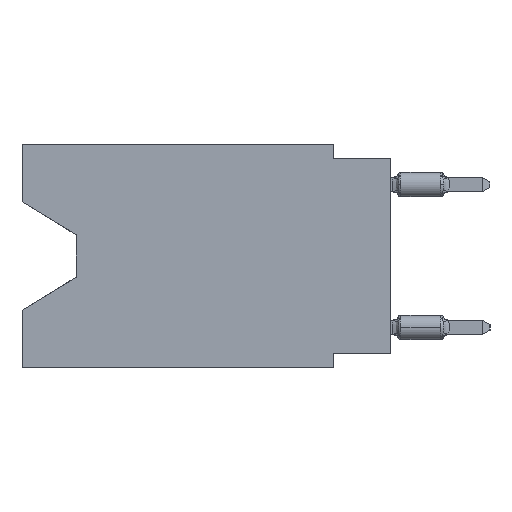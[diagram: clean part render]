
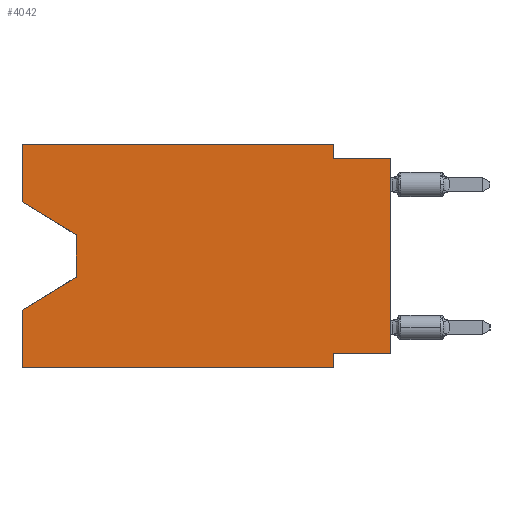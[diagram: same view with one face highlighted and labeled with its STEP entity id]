
A CAD part, left-side view. The second image highlights one B-rep face of the part: STEP entity #4042.
In plain terms, the highlighted planar face has unit normal (-1, 0, 0).
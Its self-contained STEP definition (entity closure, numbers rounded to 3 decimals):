
#632 = CARTESIAN_POINT ( 'NONE',  ( 0., 13.97, -4.013 ) ) ;
#1037 = VERTEX_POINT ( 'NONE', #12640 ) ;
#1064 = ORIENTED_EDGE ( 'NONE', *, *, #12744, .T. ) ;
#1403 = VECTOR ( 'NONE', #12382, 1000. ) ;
#1657 = LINE ( 'NONE', #27169, #15389 ) ;
#2208 = CARTESIAN_POINT ( 'NONE',  ( 0., 16.383, -7.36 ) ) ;
#2257 = VERTEX_POINT ( 'NONE', #24532 ) ;
#2273 = LINE ( 'NONE', #18485, #5044 ) ;
#2495 = VERTEX_POINT ( 'NONE', #13733 ) ;
#2797 = VERTEX_POINT ( 'NONE', #632 ) ;
#2970 = CARTESIAN_POINT ( 'NONE',  ( 0., 16.383, -2.546 ) ) ;
#3284 = VECTOR ( 'NONE', #19489, 1000. ) ;
#3533 = LINE ( 'NONE', #15798, #15662 ) ;
#3560 = DIRECTION ( 'NONE',  ( 0., 0., -1. ) ) ;
#3860 = CARTESIAN_POINT ( 'NONE',  ( 0., 2.54, -9.906 ) ) ;
#4042 = ADVANCED_FACE ( 'NONE', ( #20989 ), #18377, .F. ) ;
#4954 = CARTESIAN_POINT ( 'NONE',  ( 0., 16.383, 0. ) ) ;
#5044 = VECTOR ( 'NONE', #14252, 1000. ) ;
#5098 = CARTESIAN_POINT ( 'NONE',  ( 0., 13.97, -5.893 ) ) ;
#5673 = ORIENTED_EDGE ( 'NONE', *, *, #21150, .T. ) ;
#5781 = VECTOR ( 'NONE', #15855, 1000. ) ;
#6340 = EDGE_LOOP ( 'NONE', ( #1064, #19126, #24900, #10938, #5673, #23759, #12050, #23353, #22663, #14759, #27039, #16289 ) ) ;
#6469 = DIRECTION ( 'NONE',  ( 0., 0., 1. ) ) ;
#7064 = VECTOR ( 'NONE', #29134, 1000. ) ;
#7125 = VERTEX_POINT ( 'NONE', #28111 ) ;
#7310 = EDGE_CURVE ( 'NONE', #12395, #2495, #1657, .T. ) ;
#7480 = LINE ( 'NONE', #2970, #16596 ) ;
#8751 = CARTESIAN_POINT ( 'NONE',  ( 0., 16.383, 0. ) ) ;
#8922 = VERTEX_POINT ( 'NONE', #16013 ) ;
#9292 = DIRECTION ( 'NONE',  ( 0., 0., -1. ) ) ;
#10331 = VERTEX_POINT ( 'NONE', #26218 ) ;
#10938 = ORIENTED_EDGE ( 'NONE', *, *, #13830, .F. ) ;
#11026 = VECTOR ( 'NONE', #3560, 1000. ) ;
#11771 = CARTESIAN_POINT ( 'NONE',  ( 0., 16.383, -9.906 ) ) ;
#11910 = DIRECTION ( 'NONE',  ( 0., -0.855, -0.519 ) ) ;
#11912 = LINE ( 'NONE', #20569, #5781 ) ;
#11975 = VERTEX_POINT ( 'NONE', #26419 ) ;
#12050 = ORIENTED_EDGE ( 'NONE', *, *, #22576, .F. ) ;
#12124 = EDGE_CURVE ( 'NONE', #2257, #1037, #18767, .T. ) ;
#12382 = DIRECTION ( 'NONE',  ( 0., 0.855, -0.519 ) ) ;
#12395 = VERTEX_POINT ( 'NONE', #13130 ) ;
#12640 = CARTESIAN_POINT ( 'NONE',  ( 0., 2.54, 0. ) ) ;
#12718 = EDGE_CURVE ( 'NONE', #2797, #16454, #14493, .T. ) ;
#12744 = EDGE_CURVE ( 'NONE', #8922, #2797, #7480, .T. ) ;
#13130 = CARTESIAN_POINT ( 'NONE',  ( 0., 0., -9.271 ) ) ;
#13733 = CARTESIAN_POINT ( 'NONE',  ( 0., 0., -0.635 ) ) ;
#13830 = EDGE_CURVE ( 'NONE', #7125, #13875, #11912, .T. ) ;
#13875 = VERTEX_POINT ( 'NONE', #2208 ) ;
#14055 = LINE ( 'NONE', #11771, #3284 ) ;
#14252 = DIRECTION ( 'NONE',  ( 0., 0., -1. ) ) ;
#14493 = LINE ( 'NONE', #25759, #27319 ) ;
#14759 = ORIENTED_EDGE ( 'NONE', *, *, #25674, .F. ) ;
#14781 = DIRECTION ( 'NONE',  ( 0., 0., -1. ) ) ;
#15088 = LINE ( 'NONE', #24360, #11026 ) ;
#15389 = VECTOR ( 'NONE', #6469, 1000. ) ;
#15598 = LINE ( 'NONE', #8751, #7064 ) ;
#15662 = VECTOR ( 'NONE', #22969, 1000. ) ;
#15798 = CARTESIAN_POINT ( 'NONE',  ( 0., 0., -0.635 ) ) ;
#15855 = DIRECTION ( 'NONE',  ( 0., 0., 1. ) ) ;
#16013 = CARTESIAN_POINT ( 'NONE',  ( 0., 16.383, -2.546 ) ) ;
#16267 = DIRECTION ( 'NONE',  ( 1., 0., 0. ) ) ;
#16289 = ORIENTED_EDGE ( 'NONE', *, *, #17499, .F. ) ;
#16454 = VERTEX_POINT ( 'NONE', #16490 ) ;
#16490 = CARTESIAN_POINT ( 'NONE',  ( 0., 13.97, -5.893 ) ) ;
#16596 = VECTOR ( 'NONE', #11910, 1000. ) ;
#16630 = LINE ( 'NONE', #5098, #1403 ) ;
#17499 = EDGE_CURVE ( 'NONE', #8922, #2257, #15598, .T. ) ;
#17642 = LINE ( 'NONE', #22256, #28097 ) ;
#18377 = PLANE ( 'NONE',  #24541 ) ;
#18457 = DIRECTION ( 'NONE',  ( 0., -1., 0. ) ) ;
#18485 = CARTESIAN_POINT ( 'NONE',  ( 0., 2.54, 0. ) ) ;
#18767 = LINE ( 'NONE', #4954, #20440 ) ;
#19126 = ORIENTED_EDGE ( 'NONE', *, *, #12718, .T. ) ;
#19489 = DIRECTION ( 'NONE',  ( 0., -1., 0. ) ) ;
#20396 = DIRECTION ( 'NONE',  ( 0., 1., 0. ) ) ;
#20440 = VECTOR ( 'NONE', #18457, 1000. ) ;
#20569 = CARTESIAN_POINT ( 'NONE',  ( 0., 16.383, 0. ) ) ;
#20989 = FACE_OUTER_BOUND ( 'NONE', #6340, .T. ) ;
#21150 = EDGE_CURVE ( 'NONE', #7125, #22657, #14055, .T. ) ;
#21418 = EDGE_CURVE ( 'NONE', #11975, #22657, #15088, .T. ) ;
#22256 = CARTESIAN_POINT ( 'NONE',  ( 0., 0., -9.271 ) ) ;
#22576 = EDGE_CURVE ( 'NONE', #12395, #11975, #17642, .T. ) ;
#22657 = VERTEX_POINT ( 'NONE', #3860 ) ;
#22663 = ORIENTED_EDGE ( 'NONE', *, *, #25029, .F. ) ;
#22969 = DIRECTION ( 'NONE',  ( 0., -1., 0. ) ) ;
#23353 = ORIENTED_EDGE ( 'NONE', *, *, #7310, .T. ) ;
#23759 = ORIENTED_EDGE ( 'NONE', *, *, #21418, .F. ) ;
#24360 = CARTESIAN_POINT ( 'NONE',  ( 0., 2.54, -9.906 ) ) ;
#24532 = CARTESIAN_POINT ( 'NONE',  ( 0., 16.383, 0. ) ) ;
#24541 = AXIS2_PLACEMENT_3D ( 'NONE', #27696, #16267, #9292 ) ;
#24900 = ORIENTED_EDGE ( 'NONE', *, *, #27370, .T. ) ;
#25029 = EDGE_CURVE ( 'NONE', #10331, #2495, #3533, .T. ) ;
#25674 = EDGE_CURVE ( 'NONE', #1037, #10331, #2273, .T. ) ;
#25759 = CARTESIAN_POINT ( 'NONE',  ( 0., 13.97, -4.013 ) ) ;
#26218 = CARTESIAN_POINT ( 'NONE',  ( 0., 2.54, -0.635 ) ) ;
#26419 = CARTESIAN_POINT ( 'NONE',  ( 0., 2.54, -9.271 ) ) ;
#27039 = ORIENTED_EDGE ( 'NONE', *, *, #12124, .F. ) ;
#27169 = CARTESIAN_POINT ( 'NONE',  ( 0., 0., 0. ) ) ;
#27319 = VECTOR ( 'NONE', #14781, 1000. ) ;
#27370 = EDGE_CURVE ( 'NONE', #16454, #13875, #16630, .T. ) ;
#27696 = CARTESIAN_POINT ( 'NONE',  ( 0., 16.383, 0. ) ) ;
#28097 = VECTOR ( 'NONE', #20396, 1000. ) ;
#28111 = CARTESIAN_POINT ( 'NONE',  ( 0., 16.383, -9.906 ) ) ;
#29134 = DIRECTION ( 'NONE',  ( 0., 0., 1. ) ) ;
